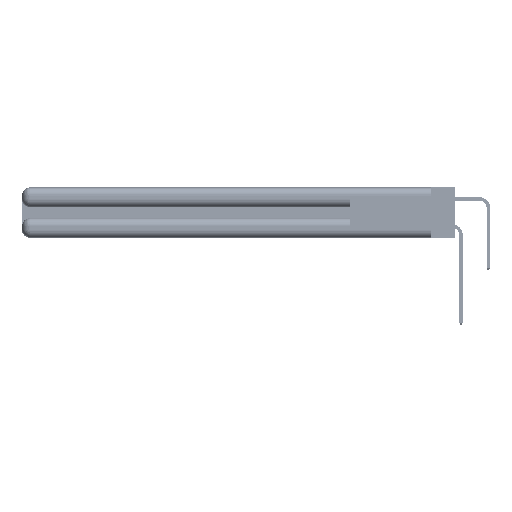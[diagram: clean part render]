
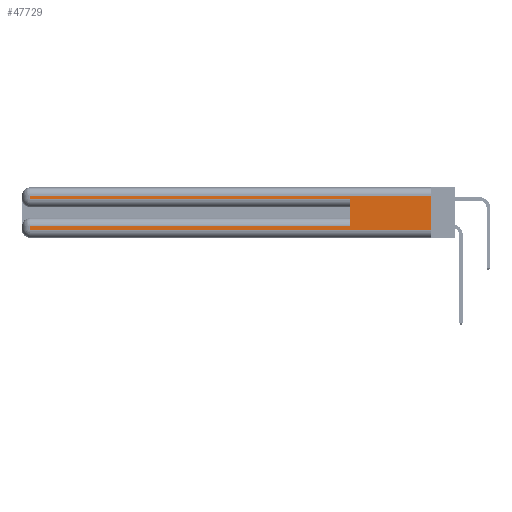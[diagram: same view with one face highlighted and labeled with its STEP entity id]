
A CAD part, left-side view. The second image highlights one B-rep face of the part: STEP entity #47729.
In plain terms, the highlighted planar face has unit normal (-1, 0, 0).
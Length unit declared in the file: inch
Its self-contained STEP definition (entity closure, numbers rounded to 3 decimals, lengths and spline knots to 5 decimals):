
#8 = VECTOR ( 'NONE', #50826, 39.37008 ) ;
#269 = DIRECTION ( 'NONE',  ( 0., 1., 0. ) ) ;
#807 = ORIENTED_EDGE ( 'NONE', *, *, #45683, .T. ) ;
#877 = ORIENTED_EDGE ( 'NONE', *, *, #26399, .T. ) ;
#1229 = LINE ( 'NONE', #29442, #34408 ) ;
#1984 = EDGE_CURVE ( 'NONE', #12503, #48758, #1229, .T. ) ;
#2593 = ORIENTED_EDGE ( 'NONE', *, *, #26481, .F. ) ;
#3400 = EDGE_CURVE ( 'NONE', #28410, #34908, #30721, .T. ) ;
#3629 = AXIS2_PLACEMENT_3D ( 'NONE', #42936, #47037, #22411 ) ;
#5264 = VECTOR ( 'NONE', #33462, 39.37008 ) ;
#5435 = CARTESIAN_POINT ( 'NONE',  ( 0., 2.94, 0.31 ) ) ;
#6301 = VERTEX_POINT ( 'NONE', #42944 ) ;
#7063 = ORIENTED_EDGE ( 'NONE', *, *, #45368, .F. ) ;
#7309 = CARTESIAN_POINT ( 'NONE',  ( 0., 0.6, 0.145 ) ) ;
#7496 = DIRECTION ( 'NONE',  ( 0., 0., 1. ) ) ;
#7503 = ORIENTED_EDGE ( 'NONE', *, *, #33361, .T. ) ;
#7679 = VECTOR ( 'NONE', #7496, 39.37008 ) ;
#8738 = EDGE_LOOP ( 'NONE', ( #2593, #19606, #19507, #7503, #7063, #43325, #807, #877 ) ) ;
#9492 = CARTESIAN_POINT ( 'NONE',  ( 0., 0., 0.37 ) ) ;
#10052 = EDGE_CURVE ( 'NONE', #34908, #42336, #38196, .T. ) ;
#10163 = CARTESIAN_POINT ( 'NONE',  ( 0., 0.6, 0.085 ) ) ;
#10215 = DIRECTION ( 'NONE',  ( 0., 0., -1. ) ) ;
#11147 = LINE ( 'NONE', #9492, #8 ) ;
#12503 = VERTEX_POINT ( 'NONE', #10163 ) ;
#14078 = PLANE ( 'NONE',  #3629 ) ;
#15140 = FACE_OUTER_BOUND ( 'NONE', #8738, .T. ) ;
#15514 = LINE ( 'NONE', #42397, #48349 ) ;
#15980 = CARTESIAN_POINT ( 'NONE',  ( 0., 0.6, 0.285 ) ) ;
#16230 = VECTOR ( 'NONE', #10215, 39.37008 ) ;
#17728 = DIRECTION ( 'NONE',  ( 0., 0., -1. ) ) ;
#19507 = ORIENTED_EDGE ( 'NONE', *, *, #10052, .T. ) ;
#19606 = ORIENTED_EDGE ( 'NONE', *, *, #3400, .T. ) ;
#22411 = DIRECTION ( 'NONE',  ( 0., 0., -1. ) ) ;
#23009 = CARTESIAN_POINT ( 'NONE',  ( 0., 0., 0.31 ) ) ;
#23507 = CARTESIAN_POINT ( 'NONE',  ( 0., 0., 0.31 ) ) ;
#25324 = CARTESIAN_POINT ( 'NONE',  ( 0., 2.94, 0.085 ) ) ;
#25356 = CARTESIAN_POINT ( 'NONE',  ( 0., 0., 0.06 ) ) ;
#26399 = EDGE_CURVE ( 'NONE', #6301, #48534, #49266, .T. ) ;
#26481 = EDGE_CURVE ( 'NONE', #28410, #48534, #11147, .T. ) ;
#28219 = CARTESIAN_POINT ( 'NONE',  ( 0., 0., 0.06 ) ) ;
#28410 = VERTEX_POINT ( 'NONE', #23507 ) ;
#29442 = CARTESIAN_POINT ( 'NONE',  ( 0., 0., 0.085 ) ) ;
#29796 = LINE ( 'NONE', #7309, #7679 ) ;
#30721 = LINE ( 'NONE', #23009, #51251 ) ;
#30918 = CARTESIAN_POINT ( 'NONE',  ( 0., 2.94, 0.37 ) ) ;
#31154 = DIRECTION ( 'NONE',  ( 0., 1., 0. ) ) ;
#32339 = CARTESIAN_POINT ( 'NONE',  ( 0., 2.94, 0.285 ) ) ;
#33361 = EDGE_CURVE ( 'NONE', #42336, #46636, #38702, .T. ) ;
#33462 = DIRECTION ( 'NONE',  ( 0., -1., 0. ) ) ;
#34408 = VECTOR ( 'NONE', #269, 39.37008 ) ;
#34908 = VERTEX_POINT ( 'NONE', #5435 ) ;
#38196 = LINE ( 'NONE', #30918, #16230 ) ;
#38702 = LINE ( 'NONE', #41111, #48286 ) ;
#41111 = CARTESIAN_POINT ( 'NONE',  ( 0., 0., 0.285 ) ) ;
#42336 = VERTEX_POINT ( 'NONE', #32339 ) ;
#42397 = CARTESIAN_POINT ( 'NONE',  ( 0., 2.94, 0.37 ) ) ;
#42936 = CARTESIAN_POINT ( 'NONE',  ( 0., 0., 0.37 ) ) ;
#42944 = CARTESIAN_POINT ( 'NONE',  ( 0., 2.94, 0.06 ) ) ;
#43325 = ORIENTED_EDGE ( 'NONE', *, *, #1984, .T. ) ;
#45229 = DIRECTION ( 'NONE',  ( 0., -1., 0. ) ) ;
#45368 = EDGE_CURVE ( 'NONE', #12503, #46636, #29796, .T. ) ;
#45683 = EDGE_CURVE ( 'NONE', #48758, #6301, #15514, .T. ) ;
#46636 = VERTEX_POINT ( 'NONE', #15980 ) ;
#47037 = DIRECTION ( 'NONE',  ( 1., 0., 0. ) ) ;
#47729 = ADVANCED_FACE ( 'NONE', ( #15140 ), #14078, .F. ) ;
#48286 = VECTOR ( 'NONE', #45229, 39.37008 ) ;
#48349 = VECTOR ( 'NONE', #17728, 39.37008 ) ;
#48534 = VERTEX_POINT ( 'NONE', #28219 ) ;
#48758 = VERTEX_POINT ( 'NONE', #25324 ) ;
#49266 = LINE ( 'NONE', #25356, #5264 ) ;
#50826 = DIRECTION ( 'NONE',  ( 0., 0., -1. ) ) ;
#51251 = VECTOR ( 'NONE', #31154, 39.37008 ) ;
